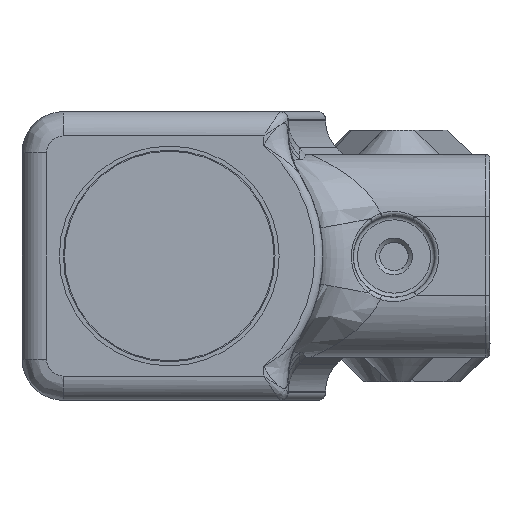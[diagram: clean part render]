
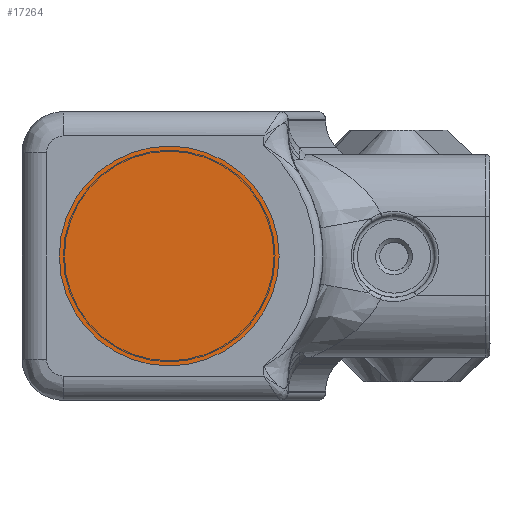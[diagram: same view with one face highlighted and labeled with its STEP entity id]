
A CAD part, left-side view. The second image highlights one B-rep face of the part: STEP entity #17264.
In plain terms, the highlighted planar face has unit normal (-1, 0, 0).
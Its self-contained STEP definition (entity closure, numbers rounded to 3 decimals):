
#526=PLANE('',#19285);
#2277=FACE_OUTER_BOUND('',#3396,.T.);
#3396=EDGE_LOOP('',(#15804));
#6575=CIRCLE('',#19284,13.5);
#8088=VERTEX_POINT('',#38458);
#10660=EDGE_CURVE('',#8088,#8088,#6575,.T.);
#15804=ORIENTED_EDGE('',*,*,#10660,.T.);
#17264=ADVANCED_FACE('',(#2277),#526,.T.);
#19284=AXIS2_PLACEMENT_3D('',#38460,#24347,#24348);
#19285=AXIS2_PLACEMENT_3D('',#38461,#24349,#24350);
#24347=DIRECTION('center_axis',(-1.,0.,0.));
#24348=DIRECTION('ref_axis',(0.,0.,
1.));
#24349=DIRECTION('center_axis',(-1.,0.,0.));
#24350=DIRECTION('ref_axis',(0.,0.,1.));
#38458=CARTESIAN_POINT('',(34.5,37.056,29.25));
#38460=CARTESIAN_POINT('Origin',(34.5,37.056,42.75));
#38461=CARTESIAN_POINT('Origin',(34.5,37.056,42.75));
